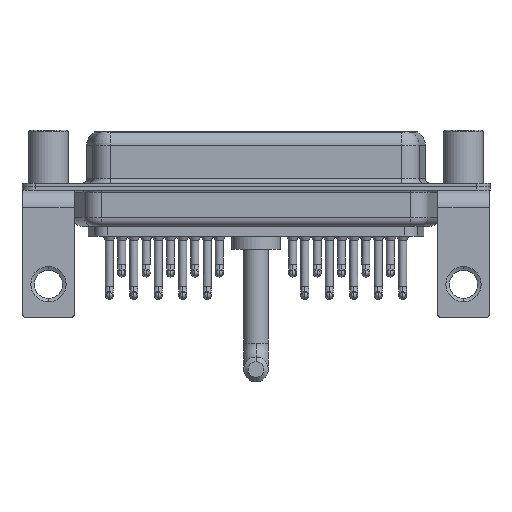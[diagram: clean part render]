
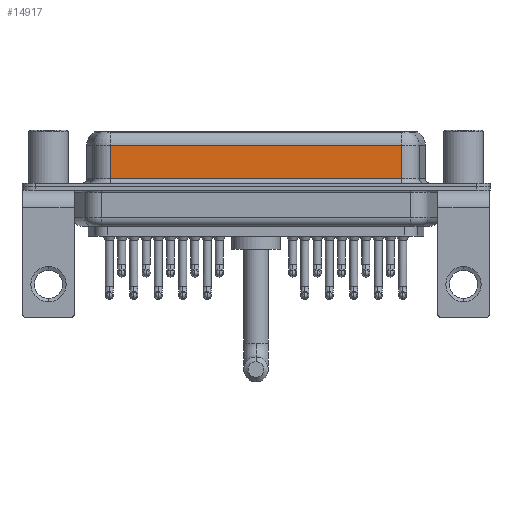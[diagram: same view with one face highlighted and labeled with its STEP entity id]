
A CAD part, front view. The second image highlights one B-rep face of the part: STEP entity #14917.
In plain terms, the highlighted planar face has unit normal (0, -1, 0).
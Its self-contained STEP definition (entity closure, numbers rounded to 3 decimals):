
#1181 = EDGE_CURVE ( 'NONE', #2475, #23272, #13441, .T. ) ;
#1612 = DIRECTION ( 'NONE',  ( 0., 0., -1. ) ) ;
#2241 = FACE_OUTER_BOUND ( 'NONE', #8463, .T. ) ;
#2475 = VERTEX_POINT ( 'NONE', #10666 ) ;
#3530 = CARTESIAN_POINT ( 'NONE',  ( 7.013, -3.95, 6.4 ) ) ;
#3698 = VECTOR ( 'NONE', #23693, 1000. ) ;
#4146 = ORIENTED_EDGE ( 'NONE', *, *, #10357, .T. ) ;
#4712 = CARTESIAN_POINT ( 'NONE',  ( 40.037, -3.95, 4.65 ) ) ;
#5731 = CARTESIAN_POINT ( 'NONE',  ( 40.037, -3.95, 0.9 ) ) ;
#6427 = CARTESIAN_POINT ( 'NONE',  ( 40.037, -3.95, 0.9 ) ) ;
#6570 = CARTESIAN_POINT ( 'NONE',  ( 7.013, -3.95, 0.9 ) ) ;
#6731 = VECTOR ( 'NONE', #1612, 1000. ) ;
#8070 = EDGE_CURVE ( 'NONE', #9594, #2475, #11737, .T. ) ;
#8463 = EDGE_LOOP ( 'NONE', ( #14605, #22139, #19576, #4146 ) ) ;
#9594 = VERTEX_POINT ( 'NONE', #4712 ) ;
#10021 = DIRECTION ( 'NONE',  ( 0., 1., 0. ) ) ;
#10357 = EDGE_CURVE ( 'NONE', #23272, #23451, #12148, .T. ) ;
#10666 = CARTESIAN_POINT ( 'NONE',  ( 7.013, -3.95, 4.65 ) ) ;
#10877 = VECTOR ( 'NONE', #24775, 1000. ) ;
#11519 = VECTOR ( 'NONE', #14171, 1000. ) ;
#11737 = LINE ( 'NONE', #15914, #3698 ) ;
#12148 = LINE ( 'NONE', #6427, #11519 ) ;
#13441 = LINE ( 'NONE', #3530, #6731 ) ;
#14171 = DIRECTION ( 'NONE',  ( 1., 0., 0. ) ) ;
#14605 = ORIENTED_EDGE ( 'NONE', *, *, #18455, .F. ) ;
#14917 = ADVANCED_FACE ( 'NONE', ( #2241 ), #15608, .F. ) ;
#15608 = PLANE ( 'NONE',  #21379 ) ;
#15914 = CARTESIAN_POINT ( 'NONE',  ( 40.037, -3.95, 4.65 ) ) ;
#17778 = DIRECTION ( 'NONE',  ( 0., 0., 1. ) ) ;
#18455 = EDGE_CURVE ( 'NONE', #9594, #23451, #21216, .T. ) ;
#19181 = CARTESIAN_POINT ( 'NONE',  ( 40.037, -3.95, 6.4 ) ) ;
#19576 = ORIENTED_EDGE ( 'NONE', *, *, #1181, .T. ) ;
#21216 = LINE ( 'NONE', #19181, #10877 ) ;
#21379 = AXIS2_PLACEMENT_3D ( 'NONE', #23394, #10021, #17778 ) ;
#22139 = ORIENTED_EDGE ( 'NONE', *, *, #8070, .T. ) ;
#23272 = VERTEX_POINT ( 'NONE', #6570 ) ;
#23394 = CARTESIAN_POINT ( 'NONE',  ( 40.037, -3.95, 6.4 ) ) ;
#23451 = VERTEX_POINT ( 'NONE', #5731 ) ;
#23693 = DIRECTION ( 'NONE',  ( -1., 0., 0. ) ) ;
#24775 = DIRECTION ( 'NONE',  ( 0., 0., -1. ) ) ;
